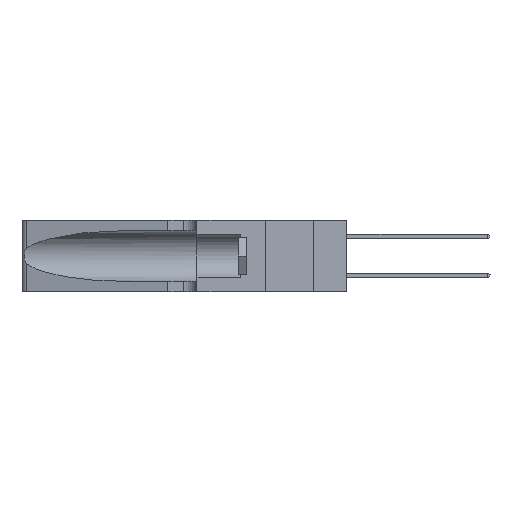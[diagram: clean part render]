
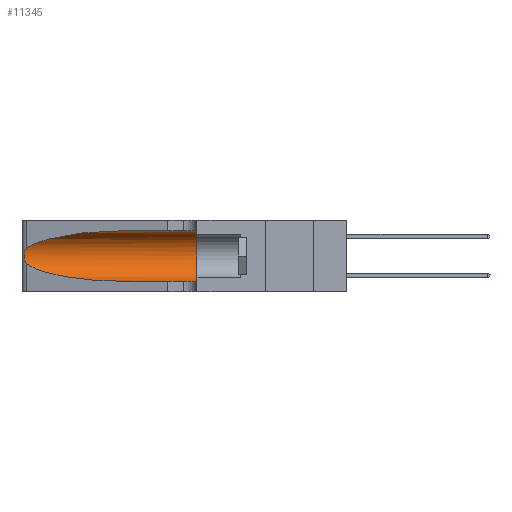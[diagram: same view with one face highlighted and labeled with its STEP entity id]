
A CAD part, left-side view. The second image highlights one B-rep face of the part: STEP entity #11345.
In plain terms, the highlighted cylindrical face has radius 3.308 mm (diameter 6.617 mm), a partial arc.
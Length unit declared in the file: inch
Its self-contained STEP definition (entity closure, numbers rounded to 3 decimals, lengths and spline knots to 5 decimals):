
#129 = VERTEX_POINT ( 'NONE', #36049 ) ;
#174 = FACE_OUTER_BOUND ( 'NONE', #20811, .T. ) ;
#177 = AXIS2_PLACEMENT_3D ( 'NONE', #21425, #4606, #24242 ) ;
#227 = CARTESIAN_POINT ( 'NONE',  ( 0.18966, 0.96281, 0.31525 ) ) ;
#794 = CARTESIAN_POINT ( 'NONE',  ( 0.26018, 1.23835, 0.19895 ) ) ;
#986 = VERTEX_POINT ( 'NONE', #9096 ) ;
#3687 = CARTESIAN_POINT ( 'NONE',  ( 0.26075, 1.23896, 0.178 ) ) ;
#3966 = ORIENTED_EDGE ( 'NONE', *, *, #17470, .T. ) ;
#3972 = CARTESIAN_POINT ( 'NONE',  ( 0.1305, 0.72297, 0.31525 ) ) ;
#4382 = LINE ( 'NONE', #12439, #10153 ) ;
#4590 = VECTOR ( 'NONE', #14089, 39.37008 ) ;
#4606 = DIRECTION ( 'NONE',  ( 0., 1., 0. ) ) ;
#6012 = CARTESIAN_POINT ( 'NONE',  ( 0.25487, 1.22718, 0.22369 ) ) ;
#6562 = CARTESIAN_POINT ( 'NONE',  ( 0.25856, 1.23593, 0.16098 ) ) ;
#7747 = DIRECTION ( 'NONE',  ( 0., 0., -1. ) ) ;
#8454 = CARTESIAN_POINT ( 'NONE',  ( 0.1305, 1.61858, 0.05475 ) ) ;
#9096 = CARTESIAN_POINT ( 'NONE',  ( 0.1305, 0.72297, 0.05475 ) ) ;
#9420 = CARTESIAN_POINT ( 'NONE',  ( 0.25639, 1.23186, 0.15144 ) ) ;
#9622 = EDGE_CURVE ( 'NONE', #24933, #129, #4382, .T. ) ;
#10153 = VECTOR ( 'NONE', #34538, 39.37008 ) ;
#10383 = ORIENTED_EDGE ( 'NONE', *, *, #15862, .T. ) ;
#10467 = EDGE_CURVE ( 'NONE', #129, #21136, #27553, .T. ) ;
#10611 = CARTESIAN_POINT ( 'NONE',  ( 0.1305, 0.72297, 0.05475 ) ) ;
#11345 = ADVANCED_FACE ( 'NONE', ( #174 ), #13531, .F. ) ;
#12101 = CARTESIAN_POINT ( 'NONE',  ( 0.25555, 1.22994, 0.2215 ) ) ;
#12236 = CARTESIAN_POINT ( 'NONE',  ( 0.25487, 1.22718, 0.14631 ) ) ;
#12439 = CARTESIAN_POINT ( 'NONE',  ( 0.1305, 1.61858, 0.31525 ) ) ;
#12925 = AXIS2_PLACEMENT_3D ( 'NONE', #32948, #16240, #7747 ) ;
#12986 = LINE ( 'NONE', #8454, #4590 ) ;
#13531 = CYLINDRICAL_SURFACE ( 'NONE', #12925, 0.13025 ) ;
#14089 = DIRECTION ( 'NONE',  ( 0., -1., 0. ) ) ;
#15109 = CARTESIAN_POINT ( 'NONE',  ( 0.25487, 1.22718, 0.22369 ) ) ;
#15151 = ORIENTED_EDGE ( 'NONE', *, *, #9622, .F. ) ;
#15862 = EDGE_CURVE ( 'NONE', #30864, #26174, #35608, .T. ) ;
#16175 =( BOUNDED_CURVE ( )  B_SPLINE_CURVE ( 3, ( #24545, #21718, #27328, #10611 ),
 .UNSPECIFIED., .F., .F. ) 
 B_SPLINE_CURVE_WITH_KNOTS ( ( 4, 4 ),
 ( 3.44316, 4.71239 ),
 .UNSPECIFIED. ) 
 CURVE ( )  GEOMETRIC_REPRESENTATION_ITEM ( )  RATIONAL_B_SPLINE_CURVE ( ( 1., 0.87, 0.87, 1. ) ) 
 REPRESENTATION_ITEM ( '' )  );
#16240 = DIRECTION ( 'NONE',  ( 0., -1., 0. ) ) ;
#17470 = EDGE_CURVE ( 'NONE', #24933, #30864, #29098, .T. ) ;
#17724 = CARTESIAN_POINT ( 'NONE',  ( 0.25854, 1.2359, 0.20912 ) ) ;
#18533 = CARTESIAN_POINT ( 'NONE',  ( 0.1305, 0.35, 0.05475 ) ) ;
#18581 = CARTESIAN_POINT ( 'NONE',  ( 0.25487, 1.22718, 0.14631 ) ) ;
#20542 = CARTESIAN_POINT ( 'NONE',  ( 0.26075, 1.23896, 0.19203 ) ) ;
#20642 = EDGE_CURVE ( 'NONE', #26174, #986, #16175, .T. ) ;
#20811 = EDGE_LOOP ( 'NONE', ( #3966, #10383, #25413, #27888, #21999, #15151 ) ) ;
#21136 = VERTEX_POINT ( 'NONE', #18533 ) ;
#21425 = CARTESIAN_POINT ( 'NONE',  ( 0.1305, 0.35, 0.185 ) ) ;
#21718 = CARTESIAN_POINT ( 'NONE',  ( 0.2373, 1.15595, 0.08982 ) ) ;
#21999 = ORIENTED_EDGE ( 'NONE', *, *, #10467, .F. ) ;
#22823 = CARTESIAN_POINT ( 'NONE',  ( 0.2373, 1.15595, 0.28018 ) ) ;
#23366 = CARTESIAN_POINT ( 'NONE',  ( 0.26017, 1.23833, 0.17102 ) ) ;
#24242 = DIRECTION ( 'NONE',  ( 0., 0., 1. ) ) ;
#24545 = CARTESIAN_POINT ( 'NONE',  ( 0.25487, 1.22718, 0.14631 ) ) ;
#24933 = VERTEX_POINT ( 'NONE', #3972 ) ;
#25267 = EDGE_CURVE ( 'NONE', #986, #21136, #12986, .T. ) ;
#25413 = ORIENTED_EDGE ( 'NONE', *, *, #20642, .T. ) ;
#26158 = CARTESIAN_POINT ( 'NONE',  ( 0.25789, 1.23486, 0.15765 ) ) ;
#26174 = VERTEX_POINT ( 'NONE', #18581 ) ;
#27328 = CARTESIAN_POINT ( 'NONE',  ( 0.18966, 0.96281, 0.05475 ) ) ;
#27553 = CIRCLE ( 'NONE', #177, 0.13025 ) ;
#27888 = ORIENTED_EDGE ( 'NONE', *, *, #25267, .T. ) ;
#28812 = CARTESIAN_POINT ( 'NONE',  ( 0.25639, 1.23184, 0.21858 ) ) ;
#28934 = CARTESIAN_POINT ( 'NONE',  ( 0.25555, 1.22993, 0.14849 ) ) ;
#29098 =( BOUNDED_CURVE ( )  B_SPLINE_CURVE ( 3, ( #31102, #227, #22823, #6012 ),
 .UNSPECIFIED., .F., .F. ) 
 B_SPLINE_CURVE_WITH_KNOTS ( ( 4, 4 ),
 ( 1.5708, 2.84003 ),
 .UNSPECIFIED. ) 
 CURVE ( )  GEOMETRIC_REPRESENTATION_ITEM ( )  RATIONAL_B_SPLINE_CURVE ( ( 1., 0.87, 0.87, 1. ) ) 
 REPRESENTATION_ITEM ( '' )  );
#30864 = VERTEX_POINT ( 'NONE', #15109 ) ;
#31102 = CARTESIAN_POINT ( 'NONE',  ( 0.1305, 0.72297, 0.31525 ) ) ;
#31626 = CARTESIAN_POINT ( 'NONE',  ( 0.25487, 1.22718, 0.22369 ) ) ;
#32948 = CARTESIAN_POINT ( 'NONE',  ( 0.1305, 1.61858, 0.185 ) ) ;
#34454 = CARTESIAN_POINT ( 'NONE',  ( 0.25787, 1.23484, 0.2124 ) ) ;
#34538 = DIRECTION ( 'NONE',  ( 0., -1., 0. ) ) ;
#35608 = B_SPLINE_CURVE_WITH_KNOTS ( 'NONE', 3,
 ( #31626, #12101, #28812, #34454, #17724, #794, #20542, #3687, #23366, #6562, #26158, #9420, #28934, #12236 ),
 .UNSPECIFIED., .F., .F.,
 ( 4, 2, 2, 2, 2, 2, 4 ),
 ( 0., 0.00027, 0.00053, 0.00107, 0.0016, 0.00187, 0.00214 ),
 .UNSPECIFIED. ) ;
#36049 = CARTESIAN_POINT ( 'NONE',  ( 0.1305, 0.35, 0.31525 ) ) ;
